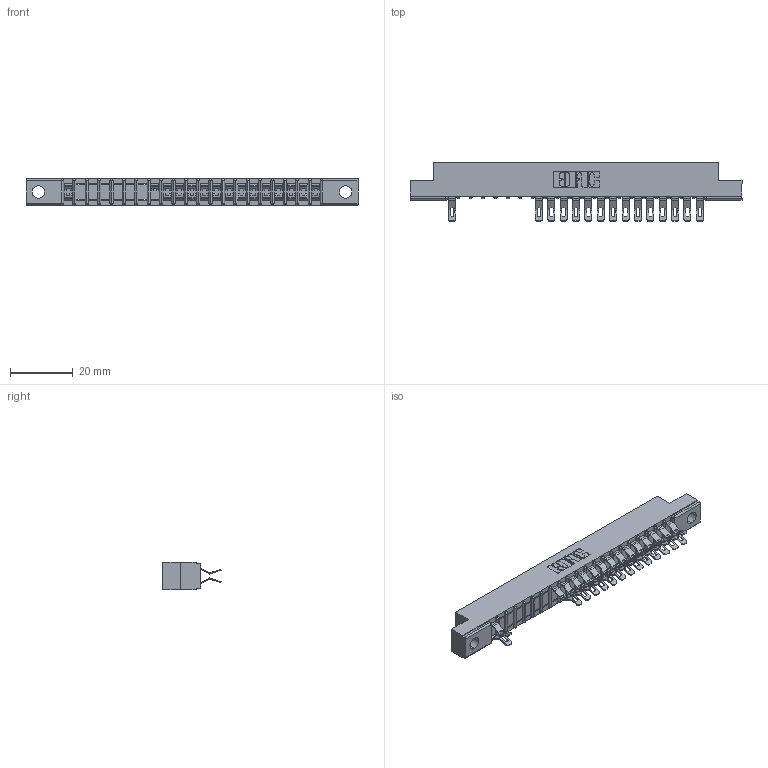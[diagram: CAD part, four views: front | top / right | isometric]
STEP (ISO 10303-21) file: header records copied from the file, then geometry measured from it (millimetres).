
FILE_DESCRIPTION (( 'STEP AP203' ), '1' );
FILE_NAME ('307-042-555-204.STEP', '2018-08-05T18:24:46', ( '' ), ( '' ), 'SwSTEP 2.0', 'SolidWorks 2016', '' );
FILE_SCHEMA (( 'CONFIG_CONTROL_DESIGN' ));
Length unit declared in the file: inch
Products named in the file (3): 307 Part_.156 Dia Mounting Holes; 307-290-001_555; 307-042-555-204
Assembly tree (30 placements, depth 2):
  307-042-555-204
    307 Part_.156 Dia Mounting Holes
    307-290-001_555  x29
Bounding box: 106.22 x 18.75 x 8.71 mm (x, y, z)
Volume: 6760.4 mm3; surface area: 11260 mm2
Topology: 30 solids, 30 shells, 2053 faces, 6024 edges, 3916 vertices
Faces by surface type: plane 1148, cylinder 861, sphere 44
Entity records: 21803 total; most frequent: CARTESIAN_POINT 3638, ORIENTED_EDGE 3616, DIRECTION 3558, EDGE_CURVE 1808, VECTOR 1374, LINE 1374, VERTEX_POINT 1172, AXIS2_PLACEMENT_3D 1092
